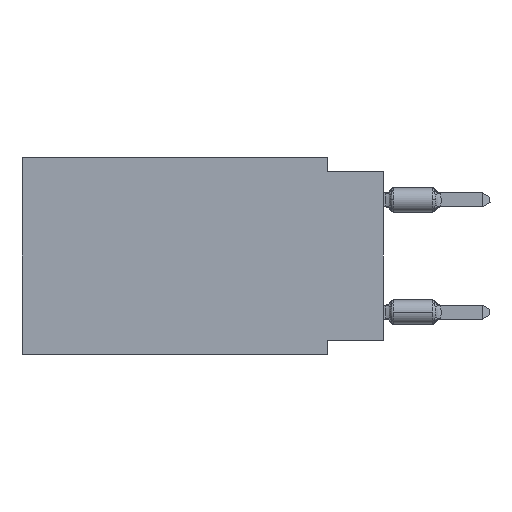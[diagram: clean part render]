
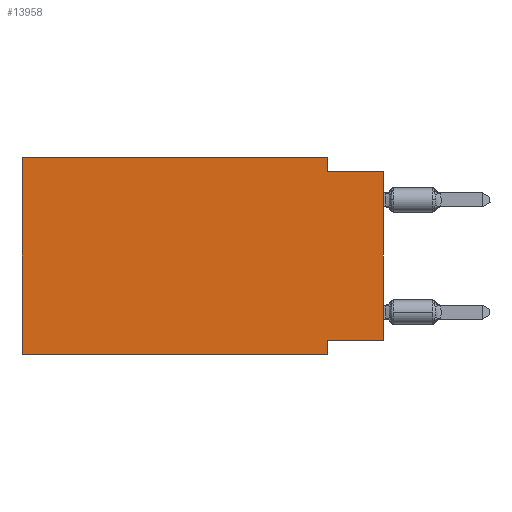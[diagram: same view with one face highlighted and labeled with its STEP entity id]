
A CAD part, left-side view. The second image highlights one B-rep face of the part: STEP entity #13958.
In plain terms, the highlighted planar face has unit normal (-1, 0, 0).
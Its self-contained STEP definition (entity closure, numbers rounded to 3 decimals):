
#855 = ORIENTED_EDGE ( 'NONE', *, *, #11303, .F. ) ;
#885 = VERTEX_POINT ( 'NONE', #3426 ) ;
#955 = CARTESIAN_POINT ( 'NONE',  ( 0., 2.54, -0.635 ) ) ;
#983 = AXIS2_PLACEMENT_3D ( 'NONE', #26237, #1628, #17896 ) ;
#991 = DIRECTION ( 'NONE',  ( 0., 0., 1. ) ) ;
#1492 = FACE_OUTER_BOUND ( 'NONE', #4247, .T. ) ;
#1500 = VECTOR ( 'NONE', #19896, 1000. ) ;
#1628 = DIRECTION ( 'NONE',  ( 1., 0., 0. ) ) ;
#1840 = CARTESIAN_POINT ( 'NONE',  ( 0., 0., -0.635 ) ) ;
#2931 = LINE ( 'NONE', #23223, #20827 ) ;
#3010 = VECTOR ( 'NONE', #991, 1000. ) ;
#3072 = VERTEX_POINT ( 'NONE', #17542 ) ;
#3191 = CARTESIAN_POINT ( 'NONE',  ( 0., 16.383, 0. ) ) ;
#3426 = CARTESIAN_POINT ( 'NONE',  ( 0., 2.54, -8.255 ) ) ;
#3523 = PLANE ( 'NONE',  #983 ) ;
#4009 = CARTESIAN_POINT ( 'NONE',  ( 0., 2.54, 0. ) ) ;
#4247 = EDGE_LOOP ( 'NONE', ( #24468, #855, #5024, #21275, #8407, #24336, #21464, #21216 ) ) ;
#4507 = EDGE_CURVE ( 'NONE', #5872, #25687, #9186, .T. ) ;
#4651 = LINE ( 'NONE', #16873, #23513 ) ;
#4936 = LINE ( 'NONE', #3191, #16449 ) ;
#5024 = ORIENTED_EDGE ( 'NONE', *, *, #7677, .F. ) ;
#5872 = VERTEX_POINT ( 'NONE', #23957 ) ;
#6920 = LINE ( 'NONE', #18871, #8934 ) ;
#7100 = CARTESIAN_POINT ( 'NONE',  ( 0., 2.54, 0. ) ) ;
#7677 = EDGE_CURVE ( 'NONE', #15867, #20991, #14090, .T. ) ;
#7952 = EDGE_CURVE ( 'NONE', #5872, #885, #2931, .T. ) ;
#8407 = ORIENTED_EDGE ( 'NONE', *, *, #22425, .F. ) ;
#8537 = DIRECTION ( 'NONE',  ( 0., -1., 0. ) ) ;
#8651 = CARTESIAN_POINT ( 'NONE',  ( 0., 0., 0. ) ) ;
#8934 = VECTOR ( 'NONE', #17108, 1000. ) ;
#9053 = VERTEX_POINT ( 'NONE', #17244 ) ;
#9186 = LINE ( 'NONE', #8651, #24971 ) ;
#11055 = VECTOR ( 'NONE', #8537, 1000. ) ;
#11303 = EDGE_CURVE ( 'NONE', #20991, #25687, #12056, .T. ) ;
#11330 = EDGE_CURVE ( 'NONE', #885, #25891, #4651, .T. ) ;
#12056 = LINE ( 'NONE', #1840, #11055 ) ;
#12711 = DIRECTION ( 'NONE',  ( 0., 0., -1. ) ) ;
#13958 = ADVANCED_FACE ( 'NONE', ( #1492 ), #3523, .F. ) ;
#14090 = LINE ( 'NONE', #4009, #1500 ) ;
#14615 = EDGE_CURVE ( 'NONE', #3072, #15867, #4936, .T. ) ;
#15867 = VERTEX_POINT ( 'NONE', #7100 ) ;
#16449 = VECTOR ( 'NONE', #23078, 1000. ) ;
#16873 = CARTESIAN_POINT ( 'NONE',  ( 0., 2.54, -8.89 ) ) ;
#17108 = DIRECTION ( 'NONE',  ( 0., -1., 0. ) ) ;
#17125 = DIRECTION ( 'NONE',  ( 0., 0., 1. ) ) ;
#17244 = CARTESIAN_POINT ( 'NONE',  ( 0., 16.383, -8.89 ) ) ;
#17300 = DIRECTION ( 'NONE',  ( 0., 1., 0. ) ) ;
#17542 = CARTESIAN_POINT ( 'NONE',  ( 0., 16.383, 0. ) ) ;
#17896 = DIRECTION ( 'NONE',  ( 0., 0., -1. ) ) ;
#18871 = CARTESIAN_POINT ( 'NONE',  ( 0., 16.383, -8.89 ) ) ;
#19791 = CARTESIAN_POINT ( 'NONE',  ( 0., 0., -0.635 ) ) ;
#19896 = DIRECTION ( 'NONE',  ( 0., 0., -1. ) ) ;
#20437 = CARTESIAN_POINT ( 'NONE',  ( 0., 2.54, -8.89 ) ) ;
#20667 = EDGE_CURVE ( 'NONE', #9053, #25891, #6920, .T. ) ;
#20827 = VECTOR ( 'NONE', #17300, 1000. ) ;
#20991 = VERTEX_POINT ( 'NONE', #955 ) ;
#21161 = LINE ( 'NONE', #25338, #3010 ) ;
#21216 = ORIENTED_EDGE ( 'NONE', *, *, #7952, .F. ) ;
#21275 = ORIENTED_EDGE ( 'NONE', *, *, #14615, .F. ) ;
#21464 = ORIENTED_EDGE ( 'NONE', *, *, #11330, .F. ) ;
#22425 = EDGE_CURVE ( 'NONE', #9053, #3072, #21161, .T. ) ;
#23078 = DIRECTION ( 'NONE',  ( 0., -1., 0. ) ) ;
#23223 = CARTESIAN_POINT ( 'NONE',  ( 0., 0., -8.255 ) ) ;
#23513 = VECTOR ( 'NONE', #12711, 1000. ) ;
#23957 = CARTESIAN_POINT ( 'NONE',  ( 0., 0., -8.255 ) ) ;
#24336 = ORIENTED_EDGE ( 'NONE', *, *, #20667, .T. ) ;
#24468 = ORIENTED_EDGE ( 'NONE', *, *, #4507, .T. ) ;
#24971 = VECTOR ( 'NONE', #17125, 1000. ) ;
#25338 = CARTESIAN_POINT ( 'NONE',  ( 0., 16.383, 0. ) ) ;
#25687 = VERTEX_POINT ( 'NONE', #19791 ) ;
#25891 = VERTEX_POINT ( 'NONE', #20437 ) ;
#26237 = CARTESIAN_POINT ( 'NONE',  ( 0., 16.383, 0. ) ) ;
